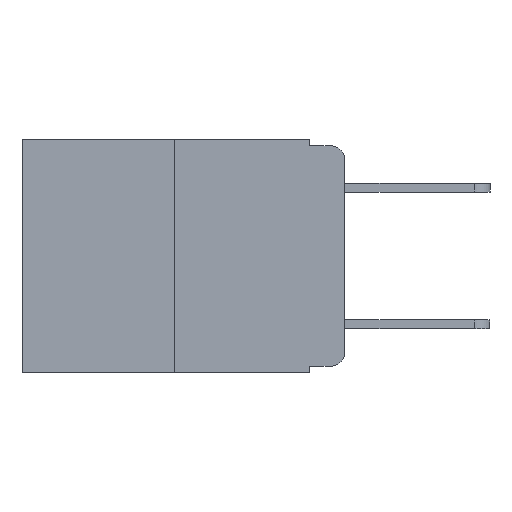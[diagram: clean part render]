
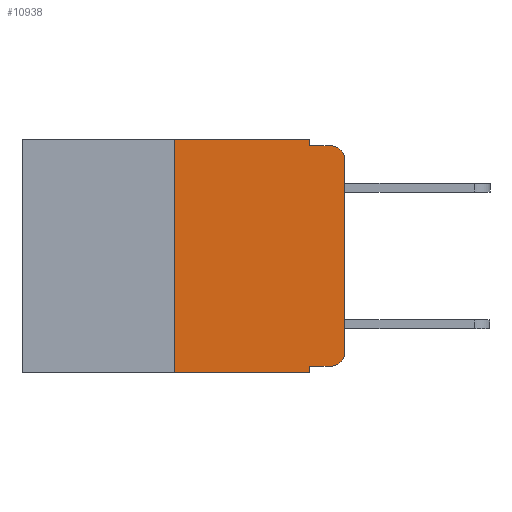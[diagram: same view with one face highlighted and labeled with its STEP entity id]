
A CAD part, left-side view. The second image highlights one B-rep face of the part: STEP entity #10938.
In plain terms, the highlighted planar face has unit normal (-1, 0, 0).
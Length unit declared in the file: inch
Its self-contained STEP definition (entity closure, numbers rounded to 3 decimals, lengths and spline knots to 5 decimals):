
#324 = ORIENTED_EDGE ( 'NONE', *, *, #4167, .F. ) ;
#325 = DIRECTION ( 'NONE',  ( 0., 0., 1. ) ) ;
#338 = ORIENTED_EDGE ( 'NONE', *, *, #3178, .F. ) ;
#464 = DIRECTION ( 'NONE',  ( 0., 0., -1. ) ) ;
#744 = DIRECTION ( 'NONE',  ( 0., -1., 0. ) ) ;
#1003 = LINE ( 'NONE', #12421, #15480 ) ;
#1191 = VERTEX_POINT ( 'NONE', #12603 ) ;
#1392 = ORIENTED_EDGE ( 'NONE', *, *, #4172, .F. ) ;
#1516 = CIRCLE ( 'NONE', #4824, 0.02 ) ;
#1592 = ORIENTED_EDGE ( 'NONE', *, *, #3790, .T. ) ;
#1862 = DIRECTION ( 'NONE',  ( 0., -1., 0. ) ) ;
#2052 = LINE ( 'NONE', #3387, #9641 ) ;
#2071 = DIRECTION ( 'NONE',  ( 0., -1., 0. ) ) ;
#3056 = ORIENTED_EDGE ( 'NONE', *, *, #4175, .F. ) ;
#3178 = EDGE_CURVE ( 'NONE', #10936, #12034, #13938, .T. ) ;
#3268 = VERTEX_POINT ( 'NONE', #11634 ) ;
#3366 = ORIENTED_EDGE ( 'NONE', *, *, #4196, .T. ) ;
#3387 = CARTESIAN_POINT ( 'NONE',  ( 0., 0., 0. ) ) ;
#3542 = VERTEX_POINT ( 'NONE', #17208 ) ;
#3739 = FACE_OUTER_BOUND ( 'NONE', #6371, .T. ) ;
#3790 = EDGE_CURVE ( 'NONE', #3268, #1191, #16621, .T. ) ;
#4120 = EDGE_CURVE ( 'NONE', #12532, #8934, #2052, .T. ) ;
#4140 = EDGE_CURVE ( 'NONE', #8934, #15888, #1516, .T. ) ;
#4141 = EDGE_CURVE ( 'NONE', #6270, #15888, #16244, .T. ) ;
#4167 = EDGE_CURVE ( 'NONE', #12034, #6270, #12525, .T. ) ;
#4172 = EDGE_CURVE ( 'NONE', #3268, #10936, #15870, .T. ) ;
#4175 = EDGE_CURVE ( 'NONE', #6654, #1191, #1003, .T. ) ;
#4196 = EDGE_CURVE ( 'NONE', #6654, #3542, #4276, .T. ) ;
#4198 = EDGE_CURVE ( 'NONE', #3542, #12532, #12109, .T. ) ;
#4276 = LINE ( 'NONE', #17349, #18168 ) ;
#4632 = CARTESIAN_POINT ( 'NONE',  ( 0., 0., -0.313 ) ) ;
#4824 = AXIS2_PLACEMENT_3D ( 'NONE', #13619, #5025, #14866 ) ;
#4867 = CARTESIAN_POINT ( 'NONE',  ( 0., 0.051, 0. ) ) ;
#4953 = DIRECTION ( 'NONE',  ( 0., 0., 1. ) ) ;
#5025 = DIRECTION ( 'NONE',  ( -1., 0., 0. ) ) ;
#5144 = DIRECTION ( 'NONE',  ( 0., 0., -1. ) ) ;
#5331 = ORIENTED_EDGE ( 'NONE', *, *, #4198, .T. ) ;
#5410 = ORIENTED_EDGE ( 'NONE', *, *, #4120, .T. ) ;
#6270 = VERTEX_POINT ( 'NONE', #7626 ) ;
#6371 = EDGE_LOOP ( 'NONE', ( #5410, #7990, #8681, #324, #338, #1392, #1592, #3056, #3366, #5331 ) ) ;
#6571 = CARTESIAN_POINT ( 'NONE',  ( 0., 0.051, 0. ) ) ;
#6654 = VERTEX_POINT ( 'NONE', #15256 ) ;
#7060 = DIRECTION ( 'NONE',  ( 0., -1., 0. ) ) ;
#7626 = CARTESIAN_POINT ( 'NONE',  ( 0., 0.051, -0.01 ) ) ;
#7990 = ORIENTED_EDGE ( 'NONE', *, *, #4140, .T. ) ;
#8102 = CARTESIAN_POINT ( 'NONE',  ( 0., 0.25, 0. ) ) ;
#8681 = ORIENTED_EDGE ( 'NONE', *, *, #4141, .F. ) ;
#8716 = VECTOR ( 'NONE', #14928, 39.37008 ) ;
#8934 = VERTEX_POINT ( 'NONE', #17874 ) ;
#9166 = VECTOR ( 'NONE', #325, 39.37008 ) ;
#9210 = DIRECTION ( 'NONE',  ( 1., 0., 0. ) ) ;
#9438 = CARTESIAN_POINT ( 'NONE',  ( 0., 0.051, -0.01 ) ) ;
#9641 = VECTOR ( 'NONE', #4953, 39.37008 ) ;
#9689 = DIRECTION ( 'NONE',  ( -1., 0., 0. ) ) ;
#10794 = AXIS2_PLACEMENT_3D ( 'NONE', #17387, #9689, #464 ) ;
#10936 = VERTEX_POINT ( 'NONE', #13381 ) ;
#10938 = ADVANCED_FACE ( 'NONE', ( #3739 ), #17046, .F. ) ;
#11430 = CARTESIAN_POINT ( 'NONE',  ( 0., 0.473, -0.343 ) ) ;
#11524 = CARTESIAN_POINT ( 'NONE',  ( 0., 0.473, 0. ) ) ;
#11634 = CARTESIAN_POINT ( 'NONE',  ( 0., 0.25, -0.343 ) ) ;
#12034 = VERTEX_POINT ( 'NONE', #4867 ) ;
#12109 = CIRCLE ( 'NONE', #10794, 0.02 ) ;
#12421 = CARTESIAN_POINT ( 'NONE',  ( 0., 0.051, 0. ) ) ;
#12525 = LINE ( 'NONE', #6571, #8716 ) ;
#12532 = VERTEX_POINT ( 'NONE', #4632 ) ;
#12603 = CARTESIAN_POINT ( 'NONE',  ( 0., 0.051, -0.343 ) ) ;
#12926 = VECTOR ( 'NONE', #1862, 39.37008 ) ;
#13356 = CARTESIAN_POINT ( 'NONE',  ( 0., 0.02, -0.01 ) ) ;
#13362 = VECTOR ( 'NONE', #744, 39.37008 ) ;
#13381 = CARTESIAN_POINT ( 'NONE',  ( 0., 0.25, 0. ) ) ;
#13619 = CARTESIAN_POINT ( 'NONE',  ( 0., 0.02, -0.03 ) ) ;
#13938 = LINE ( 'NONE', #11524, #16790 ) ;
#14642 = CARTESIAN_POINT ( 'NONE',  ( 0., 0.473, 0. ) ) ;
#14866 = DIRECTION ( 'NONE',  ( 0., 0., -1. ) ) ;
#14928 = DIRECTION ( 'NONE',  ( 0., 0., -1. ) ) ;
#15256 = CARTESIAN_POINT ( 'NONE',  ( 0., 0.051, -0.333 ) ) ;
#15480 = VECTOR ( 'NONE', #5144, 39.37008 ) ;
#15870 = LINE ( 'NONE', #8102, #9166 ) ;
#15888 = VERTEX_POINT ( 'NONE', #13356 ) ;
#16244 = LINE ( 'NONE', #9438, #12926 ) ;
#16621 = LINE ( 'NONE', #11430, #13362 ) ;
#16634 = AXIS2_PLACEMENT_3D ( 'NONE', #14642, #9210, #18149 ) ;
#16790 = VECTOR ( 'NONE', #7060, 39.37008 ) ;
#17046 = PLANE ( 'NONE',  #16634 ) ;
#17208 = CARTESIAN_POINT ( 'NONE',  ( 0., 0.02, -0.333 ) ) ;
#17349 = CARTESIAN_POINT ( 'NONE',  ( 0., 0.051, -0.333 ) ) ;
#17387 = CARTESIAN_POINT ( 'NONE',  ( 0., 0.02, -0.313 ) ) ;
#17874 = CARTESIAN_POINT ( 'NONE',  ( 0., 0., -0.03 ) ) ;
#18149 = DIRECTION ( 'NONE',  ( 0., 0., -1. ) ) ;
#18168 = VECTOR ( 'NONE', #2071, 39.37008 ) ;
